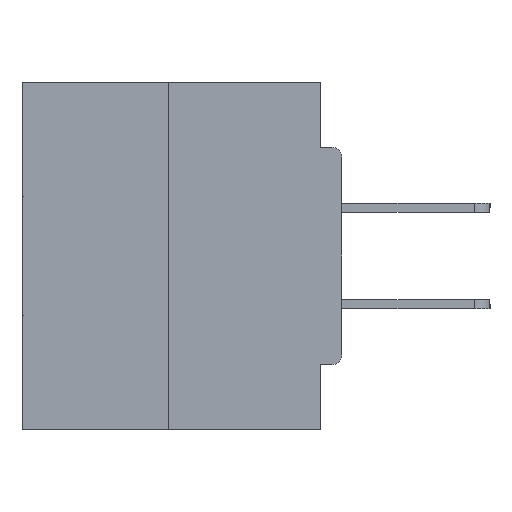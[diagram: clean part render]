
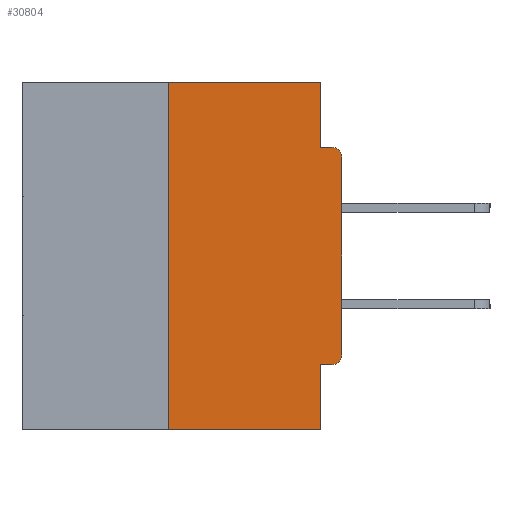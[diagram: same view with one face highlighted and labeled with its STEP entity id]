
A CAD part, left-side view. The second image highlights one B-rep face of the part: STEP entity #30804.
In plain terms, the highlighted planar face has unit normal (-1, 0, 0).
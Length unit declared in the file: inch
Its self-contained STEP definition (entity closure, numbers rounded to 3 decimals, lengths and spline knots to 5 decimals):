
#758 = CARTESIAN_POINT ( 'NONE',  ( 0., 0., -0.1085 ) ) ;
#1143 = ORIENTED_EDGE ( 'NONE', *, *, #5814, .F. ) ;
#1304 = DIRECTION ( 'NONE',  ( 0., -1., 0. ) ) ;
#1729 = CARTESIAN_POINT ( 'NONE',  ( 0., 0., 0. ) ) ;
#3869 = CARTESIAN_POINT ( 'NONE',  ( 0., 0.015, -0.0935 ) ) ;
#4395 = LINE ( 'NONE', #13641, #21656 ) ;
#4514 = DIRECTION ( 'NONE',  ( 0., 0., 1. ) ) ;
#4597 = ORIENTED_EDGE ( 'NONE', *, *, #15542, .T. ) ;
#5069 = CARTESIAN_POINT ( 'NONE',  ( 0., 0., -0.3915 ) ) ;
#5188 = VERTEX_POINT ( 'NONE', #5069 ) ;
#5372 = LINE ( 'NONE', #31012, #13758 ) ;
#5814 = EDGE_CURVE ( 'NONE', #15054, #19111, #19458, .T. ) ;
#6470 = EDGE_CURVE ( 'NONE', #32984, #15054, #9643, .T. ) ;
#7960 = VERTEX_POINT ( 'NONE', #18468 ) ;
#8141 = DIRECTION ( 'NONE',  ( 0., -1., 0. ) ) ;
#8220 = VECTOR ( 'NONE', #8141, 39.37008 ) ;
#9643 = LINE ( 'NONE', #23514, #8220 ) ;
#10248 = CIRCLE ( 'NONE', #29022, 0.015 ) ;
#10254 = VERTEX_POINT ( 'NONE', #758 ) ;
#10409 = LINE ( 'NONE', #13308, #34193 ) ;
#11063 = CARTESIAN_POINT ( 'NONE',  ( 0., 0., -0.4065 ) ) ;
#11665 = VECTOR ( 'NONE', #37954, 39.37008 ) ;
#12267 = EDGE_LOOP ( 'NONE', ( #12509, #30997, #33484, #23595, #38268, #4597, #32209, #27215, #25981, #1143 ) ) ;
#12439 = DIRECTION ( 'NONE',  ( 0., 0., -1. ) ) ;
#12509 = ORIENTED_EDGE ( 'NONE', *, *, #6470, .F. ) ;
#12652 = EDGE_CURVE ( 'NONE', #19111, #19897, #10409, .T. ) ;
#12738 = CARTESIAN_POINT ( 'NONE',  ( 0., 0.031, -0.4065 ) ) ;
#13308 = CARTESIAN_POINT ( 'NONE',  ( 0., 0., -0.0935 ) ) ;
#13587 = LINE ( 'NONE', #11063, #28552 ) ;
#13641 = CARTESIAN_POINT ( 'NONE',  ( 0., 0.46, -0.5 ) ) ;
#13758 = VECTOR ( 'NONE', #4514, 39.37008 ) ;
#14167 = CARTESIAN_POINT ( 'NONE',  ( 0., 0.25, 0. ) ) ;
#14353 = CARTESIAN_POINT ( 'NONE',  ( 0., 0.015, -0.1085 ) ) ;
#15054 = VERTEX_POINT ( 'NONE', #36844 ) ;
#15512 = EDGE_CURVE ( 'NONE', #5188, #10254, #19589, .T. ) ;
#15542 = EDGE_CURVE ( 'NONE', #15718, #5188, #10248, .T. ) ;
#15718 = VERTEX_POINT ( 'NONE', #27960 ) ;
#16346 = VERTEX_POINT ( 'NONE', #19407 ) ;
#18041 = VERTEX_POINT ( 'NONE', #12738 ) ;
#18468 = CARTESIAN_POINT ( 'NONE',  ( 0., 0.031, -0.5 ) ) ;
#18875 = FACE_OUTER_BOUND ( 'NONE', #12267, .T. ) ;
#18945 = CIRCLE ( 'NONE', #19769, 0.015 ) ;
#19111 = VERTEX_POINT ( 'NONE', #24410 ) ;
#19407 = CARTESIAN_POINT ( 'NONE',  ( 0., 0.25, -0.5 ) ) ;
#19458 = LINE ( 'NONE', #21170, #26033 ) ;
#19589 = LINE ( 'NONE', #1729, #11665 ) ;
#19769 = AXIS2_PLACEMENT_3D ( 'NONE', #14353, #26374, #31990 ) ;
#19897 = VERTEX_POINT ( 'NONE', #3869 ) ;
#20066 = EDGE_CURVE ( 'NONE', #18041, #7960, #31969, .T. ) ;
#20374 = DIRECTION ( 'NONE',  ( 0., 0., -1. ) ) ;
#20526 = CARTESIAN_POINT ( 'NONE',  ( 0., 0.46, 0. ) ) ;
#21170 = CARTESIAN_POINT ( 'NONE',  ( 0., 0.031, 0. ) ) ;
#21656 = VECTOR ( 'NONE', #37628, 39.37008 ) ;
#23514 = CARTESIAN_POINT ( 'NONE',  ( 0., 0.46, 0. ) ) ;
#23530 = DIRECTION ( 'NONE',  ( 1., 0., 0. ) ) ;
#23595 = ORIENTED_EDGE ( 'NONE', *, *, #20066, .F. ) ;
#24410 = CARTESIAN_POINT ( 'NONE',  ( 0., 0.031, -0.0935 ) ) ;
#25594 = CARTESIAN_POINT ( 'NONE',  ( 0., 0.031, -0.5 ) ) ;
#25981 = ORIENTED_EDGE ( 'NONE', *, *, #12652, .F. ) ;
#26033 = VECTOR ( 'NONE', #12439, 39.37008 ) ;
#26260 = CARTESIAN_POINT ( 'NONE',  ( 0., 0.015, -0.3915 ) ) ;
#26374 = DIRECTION ( 'NONE',  ( -1., 0., 0. ) ) ;
#27215 = ORIENTED_EDGE ( 'NONE', *, *, #29288, .T. ) ;
#27960 = CARTESIAN_POINT ( 'NONE',  ( 0., 0.015, -0.4065 ) ) ;
#28552 = VECTOR ( 'NONE', #31941, 39.37008 ) ;
#29022 = AXIS2_PLACEMENT_3D ( 'NONE', #26260, #38225, #20374 ) ;
#29037 = DIRECTION ( 'NONE',  ( 0., 0., -1. ) ) ;
#29178 = VECTOR ( 'NONE', #31736, 39.37008 ) ;
#29288 = EDGE_CURVE ( 'NONE', #10254, #19897, #18945, .T. ) ;
#30264 = EDGE_CURVE ( 'NONE', #16346, #32984, #5372, .T. ) ;
#30339 = AXIS2_PLACEMENT_3D ( 'NONE', #20526, #23530, #29037 ) ;
#30804 = ADVANCED_FACE ( 'NONE', ( #18875 ), #35211, .F. ) ;
#30997 = ORIENTED_EDGE ( 'NONE', *, *, #30264, .F. ) ;
#31012 = CARTESIAN_POINT ( 'NONE',  ( 0., 0.25, 0. ) ) ;
#31182 = EDGE_CURVE ( 'NONE', #16346, #7960, #4395, .T. ) ;
#31736 = DIRECTION ( 'NONE',  ( 0., 0., -1. ) ) ;
#31941 = DIRECTION ( 'NONE',  ( 0., 1., 0. ) ) ;
#31969 = LINE ( 'NONE', #25594, #29178 ) ;
#31990 = DIRECTION ( 'NONE',  ( 0., 0., -1. ) ) ;
#32209 = ORIENTED_EDGE ( 'NONE', *, *, #15512, .T. ) ;
#32966 = EDGE_CURVE ( 'NONE', #15718, #18041, #13587, .T. ) ;
#32984 = VERTEX_POINT ( 'NONE', #14167 ) ;
#33484 = ORIENTED_EDGE ( 'NONE', *, *, #31182, .T. ) ;
#34193 = VECTOR ( 'NONE', #1304, 39.37008 ) ;
#35211 = PLANE ( 'NONE',  #30339 ) ;
#36844 = CARTESIAN_POINT ( 'NONE',  ( 0., 0.031, 0. ) ) ;
#37628 = DIRECTION ( 'NONE',  ( 0., -1., 0. ) ) ;
#37954 = DIRECTION ( 'NONE',  ( 0., 0., 1. ) ) ;
#38225 = DIRECTION ( 'NONE',  ( -1., 0., 0. ) ) ;
#38268 = ORIENTED_EDGE ( 'NONE', *, *, #32966, .F. ) ;
